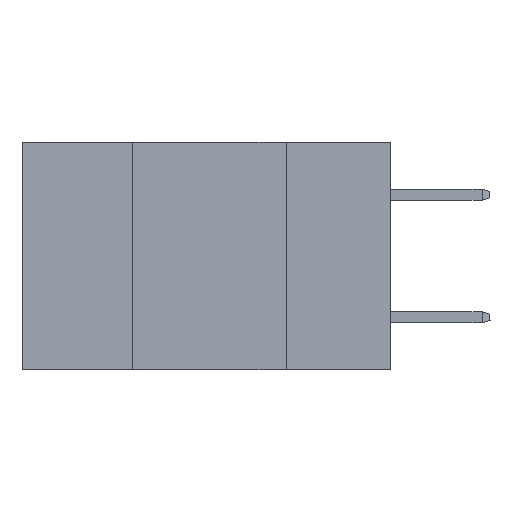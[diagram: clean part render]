
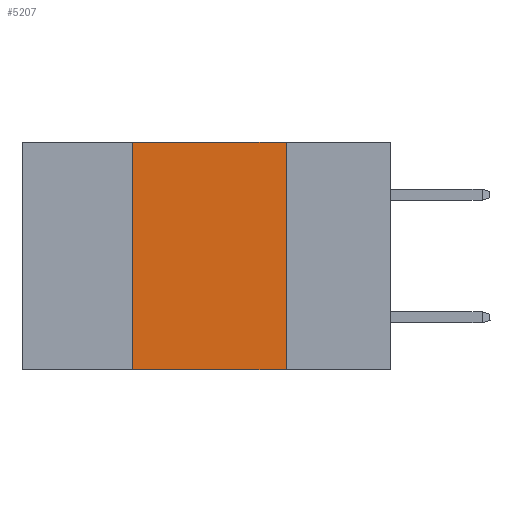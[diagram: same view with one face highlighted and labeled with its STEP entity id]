
A CAD part, left-side view. The second image highlights one B-rep face of the part: STEP entity #5207.
In plain terms, the highlighted planar face has unit normal (-1, 0, 0).
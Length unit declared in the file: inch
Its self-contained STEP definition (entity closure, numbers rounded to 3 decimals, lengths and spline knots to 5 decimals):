
#1490 = DIRECTION ( 'NONE',  ( 0., 0., 1. ) ) ;
#1637 = VERTEX_POINT ( 'NONE', #5708 ) ;
#1733 = CARTESIAN_POINT ( 'NONE',  ( 0., 0.6, 0. ) ) ;
#2111 = CARTESIAN_POINT ( 'NONE',  ( 0., 0.42, 0. ) ) ;
#2126 = ORIENTED_EDGE ( 'NONE', *, *, #11323, .T. ) ;
#2552 = DIRECTION ( 'NONE',  ( 1., 0., 0. ) ) ;
#2630 = PLANE ( 'NONE',  #5844 ) ;
#3605 = DIRECTION ( 'NONE',  ( 0., 0., -1. ) ) ;
#3669 = VECTOR ( 'NONE', #1490, 39.37008 ) ;
#4430 = DIRECTION ( 'NONE',  ( 0., 0., -1. ) ) ;
#4616 = EDGE_CURVE ( 'NONE', #5106, #1637, #8060, .T. ) ;
#5036 = CARTESIAN_POINT ( 'NONE',  ( 0., 0.42, 0. ) ) ;
#5106 = VERTEX_POINT ( 'NONE', #9748 ) ;
#5207 = ADVANCED_FACE ( 'NONE', ( #8194 ), #2630, .F. ) ;
#5307 = VERTEX_POINT ( 'NONE', #5460 ) ;
#5326 = LINE ( 'NONE', #5036, #3669 ) ;
#5350 = DIRECTION ( 'NONE',  ( 0., -1., 0. ) ) ;
#5460 = CARTESIAN_POINT ( 'NONE',  ( 0., 0.42, -0.37 ) ) ;
#5657 = VECTOR ( 'NONE', #10475, 39.37008 ) ;
#5708 = CARTESIAN_POINT ( 'NONE',  ( 0., 0.17, -0.37 ) ) ;
#5793 = EDGE_LOOP ( 'NONE', ( #10031, #6202, #5828, #2126 ) ) ;
#5828 = ORIENTED_EDGE ( 'NONE', *, *, #7634, .F. ) ;
#5844 = AXIS2_PLACEMENT_3D ( 'NONE', #1733, #2552, #3605 ) ;
#6202 = ORIENTED_EDGE ( 'NONE', *, *, #11096, .F. ) ;
#6932 = CARTESIAN_POINT ( 'NONE',  ( 0., 0.6, -0.37 ) ) ;
#7634 = EDGE_CURVE ( 'NONE', #5307, #8804, #5326, .T. ) ;
#8060 = LINE ( 'NONE', #9797, #9619 ) ;
#8194 = FACE_OUTER_BOUND ( 'NONE', #5793, .T. ) ;
#8310 = LINE ( 'NONE', #6932, #5657 ) ;
#8804 = VERTEX_POINT ( 'NONE', #2111 ) ;
#9318 = VECTOR ( 'NONE', #5350, 39.37008 ) ;
#9619 = VECTOR ( 'NONE', #4430, 39.37008 ) ;
#9720 = LINE ( 'NONE', #11500, #9318 ) ;
#9748 = CARTESIAN_POINT ( 'NONE',  ( 0., 0.17, 0. ) ) ;
#9797 = CARTESIAN_POINT ( 'NONE',  ( 0., 0.17, 0. ) ) ;
#10031 = ORIENTED_EDGE ( 'NONE', *, *, #4616, .F. ) ;
#10475 = DIRECTION ( 'NONE',  ( 0., -1., 0. ) ) ;
#11096 = EDGE_CURVE ( 'NONE', #8804, #5106, #9720, .T. ) ;
#11323 = EDGE_CURVE ( 'NONE', #5307, #1637, #8310, .T. ) ;
#11500 = CARTESIAN_POINT ( 'NONE',  ( 0., 0.6, 0. ) ) ;
